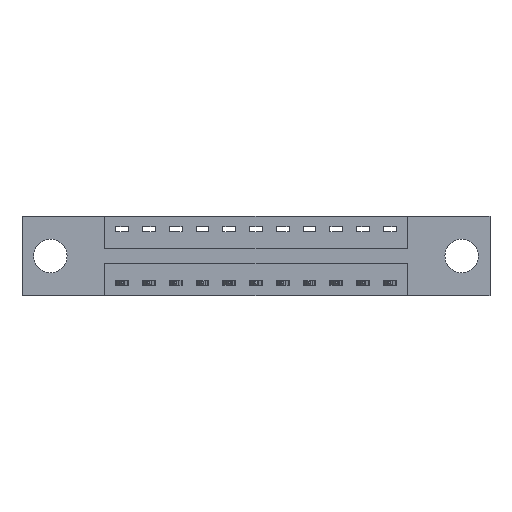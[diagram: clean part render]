
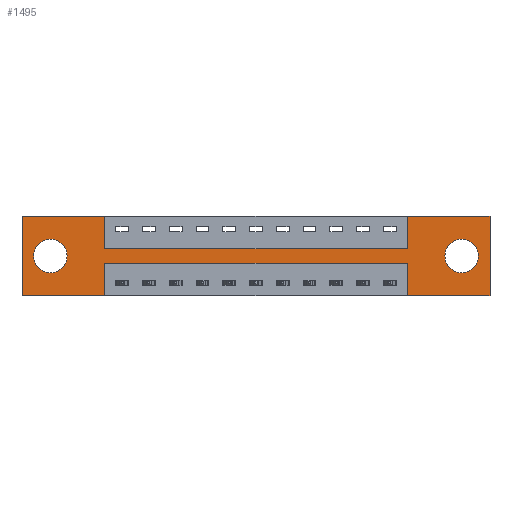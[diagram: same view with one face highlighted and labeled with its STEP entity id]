
A CAD part, front view. The second image highlights one B-rep face of the part: STEP entity #1495.
In plain terms, the highlighted planar face has unit normal (0, -1, 0).
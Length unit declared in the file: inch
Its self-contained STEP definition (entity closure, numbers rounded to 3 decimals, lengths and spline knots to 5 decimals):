
#17 = VERTEX_POINT ( 'NONE', #6451 ) ;
#35 = CARTESIAN_POINT ( 'NONE',  ( 0., 0., 0. ) ) ;
#51 = VERTEX_POINT ( 'NONE', #1335 ) ;
#152 = LINE ( 'NONE', #5672, #5906 ) ;
#310 = CARTESIAN_POINT ( 'NONE',  ( 1.7975, 0., -0.22 ) ) ;
#323 = DIRECTION ( 'NONE',  ( 0., 0., -1. ) ) ;
#385 = EDGE_CURVE ( 'NONE', #2860, #10396, #4417, .T. ) ;
#411 = VECTOR ( 'NONE', #10143, 39.37008 ) ;
#446 = LINE ( 'NONE', #7504, #8176 ) ;
#583 = CARTESIAN_POINT ( 'NONE',  ( 0.1325, 0., -0.107 ) ) ;
#653 = EDGE_CURVE ( 'NONE', #4988, #8532, #8286, .T. ) ;
#667 = LINE ( 'NONE', #9063, #1839 ) ;
#741 = ORIENTED_EDGE ( 'NONE', *, *, #8437, .F. ) ;
#791 = CARTESIAN_POINT ( 'NONE',  ( 2.185, 0., -0.37 ) ) ;
#1121 = DIRECTION ( 'NONE',  ( 0., 1., 0. ) ) ;
#1335 = CARTESIAN_POINT ( 'NONE',  ( 1.7975, 0., -0.15 ) ) ;
#1407 = CARTESIAN_POINT ( 'NONE',  ( 2.0525, 0., -0.263 ) ) ;
#1459 = CARTESIAN_POINT ( 'NONE',  ( 0.1325, 0., -0.185 ) ) ;
#1478 = AXIS2_PLACEMENT_3D ( 'NONE', #7275, #3784, #8895 ) ;
#1495 = ADVANCED_FACE ( 'NONE', ( #10897, #1972, #7712 ), #7326, .T. ) ;
#1504 = ORIENTED_EDGE ( 'NONE', *, *, #7292, .F. ) ;
#1674 = CIRCLE ( 'NONE', #2894, 0.078 ) ;
#1772 = LINE ( 'NONE', #8394, #10706 ) ;
#1839 = VECTOR ( 'NONE', #8312, 39.37008 ) ;
#1972 = FACE_BOUND ( 'NONE', #9969, .T. ) ;
#2160 = CARTESIAN_POINT ( 'NONE',  ( 0.3875, 0., 0. ) ) ;
#2187 = AXIS2_PLACEMENT_3D ( 'NONE', #6962, #4401, #7824 ) ;
#2242 = CARTESIAN_POINT ( 'NONE',  ( 0.3875, 0., -0.37 ) ) ;
#2253 = DIRECTION ( 'NONE',  ( 0., -1., 0. ) ) ;
#2266 = EDGE_CURVE ( 'NONE', #7266, #6655, #1772, .T. ) ;
#2283 = ORIENTED_EDGE ( 'NONE', *, *, #2694, .F. ) ;
#2299 = VECTOR ( 'NONE', #8200, 39.37008 ) ;
#2336 = CARTESIAN_POINT ( 'NONE',  ( 0., 0., -0.37 ) ) ;
#2402 = DIRECTION ( 'NONE',  ( -1., 0., 0. ) ) ;
#2444 = CARTESIAN_POINT ( 'NONE',  ( 2.185, 0., 0. ) ) ;
#2602 = DIRECTION ( 'NONE',  ( 0., 0., 1. ) ) ;
#2694 = EDGE_CURVE ( 'NONE', #3565, #4742, #10803, .T. ) ;
#2774 = ORIENTED_EDGE ( 'NONE', *, *, #2266, .F. ) ;
#2860 = VERTEX_POINT ( 'NONE', #6552 ) ;
#2866 = EDGE_CURVE ( 'NONE', #9657, #4988, #3326, .T. ) ;
#2894 = AXIS2_PLACEMENT_3D ( 'NONE', #10466, #1121, #323 ) ;
#3126 = DIRECTION ( 'NONE',  ( -1., 0., 0. ) ) ;
#3226 = CIRCLE ( 'NONE', #1478, 0.078 ) ;
#3318 = DIRECTION ( 'NONE',  ( 0., 0., 1. ) ) ;
#3326 = LINE ( 'NONE', #2336, #7721 ) ;
#3565 = VERTEX_POINT ( 'NONE', #2444 ) ;
#3716 = ORIENTED_EDGE ( 'NONE', *, *, #5297, .F. ) ;
#3784 = DIRECTION ( 'NONE',  ( 0., 1., 0. ) ) ;
#3859 = CARTESIAN_POINT ( 'NONE',  ( 1.7975, 0., 0. ) ) ;
#3936 = CARTESIAN_POINT ( 'NONE',  ( 0., 0., -0.37 ) ) ;
#4401 = DIRECTION ( 'NONE',  ( 0., 1., 0. ) ) ;
#4417 = LINE ( 'NONE', #2160, #2299 ) ;
#4532 = ORIENTED_EDGE ( 'NONE', *, *, #7711, .T. ) ;
#4536 = LINE ( 'NONE', #9259, #411 ) ;
#4570 = ORIENTED_EDGE ( 'NONE', *, *, #2866, .F. ) ;
#4667 = EDGE_CURVE ( 'NONE', #6342, #17, #7218, .T. ) ;
#4698 = VERTEX_POINT ( 'NONE', #7715 ) ;
#4709 = EDGE_CURVE ( 'NONE', #8828, #3565, #4536, .T. ) ;
#4742 = VERTEX_POINT ( 'NONE', #791 ) ;
#4781 = DIRECTION ( 'NONE',  ( 0., 0., -1. ) ) ;
#4802 = CARTESIAN_POINT ( 'NONE',  ( 1.7975, 0., -0.37 ) ) ;
#4929 = CARTESIAN_POINT ( 'NONE',  ( 0.3875, 0., -0.37 ) ) ;
#4938 = VECTOR ( 'NONE', #10736, 39.37008 ) ;
#4988 = VERTEX_POINT ( 'NONE', #6419 ) ;
#5201 = DIRECTION ( 'NONE',  ( 0., 0., 1. ) ) ;
#5297 = EDGE_CURVE ( 'NONE', #51, #8828, #6095, .T. ) ;
#5579 = VECTOR ( 'NONE', #6714, 39.37008 ) ;
#5672 = CARTESIAN_POINT ( 'NONE',  ( 0., 0., 0. ) ) ;
#5772 = EDGE_CURVE ( 'NONE', #4698, #9657, #8371, .T. ) ;
#5884 = EDGE_LOOP ( 'NONE', ( #8662, #1504, #2774, #741, #2283, #9930, #3716, #10058, #5961, #7968, #8974, #4570 ) ) ;
#5906 = VECTOR ( 'NONE', #10655, 39.37008 ) ;
#5917 = VECTOR ( 'NONE', #10243, 39.37008 ) ;
#5961 = ORIENTED_EDGE ( 'NONE', *, *, #385, .F. ) ;
#6095 = LINE ( 'NONE', #10865, #8091 ) ;
#6342 = VERTEX_POINT ( 'NONE', #583 ) ;
#6419 = CARTESIAN_POINT ( 'NONE',  ( 0., 0., -0.37 ) ) ;
#6451 = CARTESIAN_POINT ( 'NONE',  ( 0.1325, 0., -0.263 ) ) ;
#6552 = CARTESIAN_POINT ( 'NONE',  ( 0.3875, 0., 0. ) ) ;
#6655 = VERTEX_POINT ( 'NONE', #310 ) ;
#6707 = LINE ( 'NONE', #7645, #5917 ) ;
#6714 = DIRECTION ( 'NONE',  ( 0., 0., -1. ) ) ;
#6893 = CIRCLE ( 'NONE', #2187, 0.078 ) ;
#6962 = CARTESIAN_POINT ( 'NONE',  ( 2.0525, 0., -0.185 ) ) ;
#7218 = CIRCLE ( 'NONE', #7921, 0.078 ) ;
#7266 = VERTEX_POINT ( 'NONE', #4802 ) ;
#7275 = CARTESIAN_POINT ( 'NONE',  ( 0.1325, 0., -0.185 ) ) ;
#7292 = EDGE_CURVE ( 'NONE', #6655, #4698, #667, .T. ) ;
#7326 = PLANE ( 'NONE',  #9513 ) ;
#7504 = CARTESIAN_POINT ( 'NONE',  ( 0., 0., -0.37 ) ) ;
#7645 = CARTESIAN_POINT ( 'NONE',  ( 0.3875, 0., -0.15 ) ) ;
#7711 = EDGE_CURVE ( 'NONE', #10804, #10183, #1674, .T. ) ;
#7712 = FACE_OUTER_BOUND ( 'NONE', #5884, .T. ) ;
#7715 = CARTESIAN_POINT ( 'NONE',  ( 0.3875, 0., -0.22 ) ) ;
#7721 = VECTOR ( 'NONE', #3126, 39.37008 ) ;
#7819 = EDGE_CURVE ( 'NONE', #8532, #2860, #152, .T. ) ;
#7824 = DIRECTION ( 'NONE',  ( 0., 0., -1. ) ) ;
#7921 = AXIS2_PLACEMENT_3D ( 'NONE', #1459, #10275, #2602 ) ;
#7968 = ORIENTED_EDGE ( 'NONE', *, *, #7819, .F. ) ;
#8091 = VECTOR ( 'NONE', #5201, 39.37008 ) ;
#8176 = VECTOR ( 'NONE', #2402, 39.37008 ) ;
#8187 = CARTESIAN_POINT ( 'NONE',  ( 2.185, 0., 0. ) ) ;
#8200 = DIRECTION ( 'NONE',  ( 0., 0., -1. ) ) ;
#8286 = LINE ( 'NONE', #8670, #10271 ) ;
#8312 = DIRECTION ( 'NONE',  ( -1., 0., 0. ) ) ;
#8371 = LINE ( 'NONE', #4929, #5579 ) ;
#8394 = CARTESIAN_POINT ( 'NONE',  ( 1.7975, 0., -0.37 ) ) ;
#8437 = EDGE_CURVE ( 'NONE', #4742, #7266, #446, .T. ) ;
#8519 = EDGE_CURVE ( 'NONE', #10396, #51, #6707, .T. ) ;
#8532 = VERTEX_POINT ( 'NONE', #35 ) ;
#8662 = ORIENTED_EDGE ( 'NONE', *, *, #5772, .F. ) ;
#8670 = CARTESIAN_POINT ( 'NONE',  ( 0., 0., 0. ) ) ;
#8828 = VERTEX_POINT ( 'NONE', #3859 ) ;
#8895 = DIRECTION ( 'NONE',  ( 0., 0., 1. ) ) ;
#8974 = ORIENTED_EDGE ( 'NONE', *, *, #653, .F. ) ;
#9063 = CARTESIAN_POINT ( 'NONE',  ( 0.3875, 0., -0.22 ) ) ;
#9259 = CARTESIAN_POINT ( 'NONE',  ( 0., 0., 0. ) ) ;
#9328 = EDGE_CURVE ( 'NONE', #10183, #10804, #6893, .T. ) ;
#9513 = AXIS2_PLACEMENT_3D ( 'NONE', #3936, #2253, #4781 ) ;
#9644 = CARTESIAN_POINT ( 'NONE',  ( 2.0525, 0., -0.107 ) ) ;
#9657 = VERTEX_POINT ( 'NONE', #2242 ) ;
#9773 = ORIENTED_EDGE ( 'NONE', *, *, #4667, .T. ) ;
#9930 = ORIENTED_EDGE ( 'NONE', *, *, #4709, .F. ) ;
#9969 = EDGE_LOOP ( 'NONE', ( #9773, #10141 ) ) ;
#10053 = CARTESIAN_POINT ( 'NONE',  ( 0.3875, 0., -0.15 ) ) ;
#10058 = ORIENTED_EDGE ( 'NONE', *, *, #8519, .F. ) ;
#10141 = ORIENTED_EDGE ( 'NONE', *, *, #11034, .T. ) ;
#10143 = DIRECTION ( 'NONE',  ( 1., 0., 0. ) ) ;
#10183 = VERTEX_POINT ( 'NONE', #1407 ) ;
#10243 = DIRECTION ( 'NONE',  ( 1., 0., 0. ) ) ;
#10271 = VECTOR ( 'NONE', #10407, 39.37008 ) ;
#10275 = DIRECTION ( 'NONE',  ( 0., 1., 0. ) ) ;
#10396 = VERTEX_POINT ( 'NONE', #10053 ) ;
#10407 = DIRECTION ( 'NONE',  ( 0., 0., 1. ) ) ;
#10443 = EDGE_LOOP ( 'NONE', ( #4532, #10570 ) ) ;
#10466 = CARTESIAN_POINT ( 'NONE',  ( 2.0525, 0., -0.185 ) ) ;
#10570 = ORIENTED_EDGE ( 'NONE', *, *, #9328, .T. ) ;
#10655 = DIRECTION ( 'NONE',  ( 1., 0., 0. ) ) ;
#10706 = VECTOR ( 'NONE', #3318, 39.37008 ) ;
#10736 = DIRECTION ( 'NONE',  ( 0., 0., -1. ) ) ;
#10803 = LINE ( 'NONE', #8187, #4938 ) ;
#10804 = VERTEX_POINT ( 'NONE', #9644 ) ;
#10865 = CARTESIAN_POINT ( 'NONE',  ( 1.7975, 0., 0. ) ) ;
#10897 = FACE_BOUND ( 'NONE', #10443, .T. ) ;
#11034 = EDGE_CURVE ( 'NONE', #17, #6342, #3226, .T. ) ;
